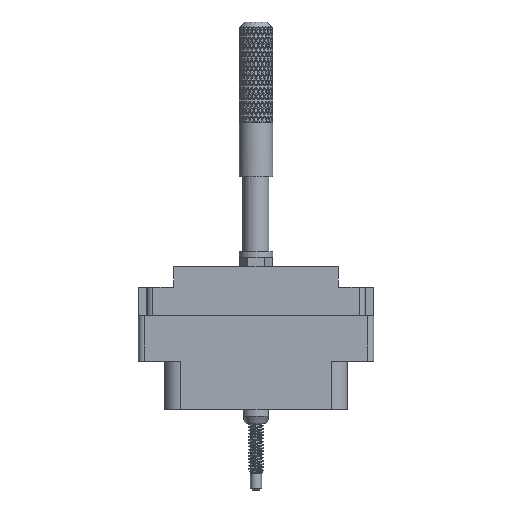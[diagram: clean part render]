
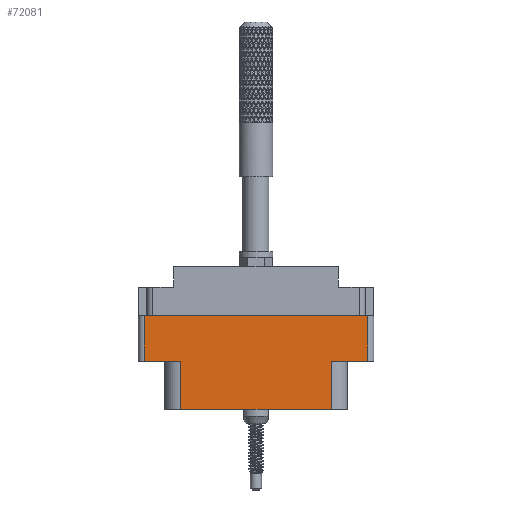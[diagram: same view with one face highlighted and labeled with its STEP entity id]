
A CAD part, front view. The second image highlights one B-rep face of the part: STEP entity #72081.
In plain terms, the highlighted planar face has unit normal (0, -1, 0).
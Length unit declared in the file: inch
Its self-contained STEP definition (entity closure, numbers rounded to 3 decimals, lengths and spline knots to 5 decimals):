
#5053 = CARTESIAN_POINT ( 'NONE',  ( -0.624, -0.343, -0.798 ) ) ;
#5832 = CARTESIAN_POINT ( 'NONE',  ( 0., -0.343, -0.274 ) ) ;
#7394 = ORIENTED_EDGE ( 'NONE', *, *, #25610, .T. ) ;
#9197 = DIRECTION ( 'NONE',  ( 0., 0., 1. ) ) ;
#9800 = CARTESIAN_POINT ( 'NONE',  ( 0.42052, -0.343, -0.529 ) ) ;
#10342 = EDGE_CURVE ( 'NONE', #183956, #45359, #106968, .T. ) ;
#12614 = VERTEX_POINT ( 'NONE', #67093 ) ;
#13844 = EDGE_LOOP ( 'NONE', ( #74284, #50483, #7394, #42640, #83809, #131305, #63630, #53074 ) ) ;
#14874 = CARTESIAN_POINT ( 'NONE',  ( -0.624, -0.343, -0.529 ) ) ;
#17578 = VECTOR ( 'NONE', #175656, 39.37008 ) ;
#25610 = EDGE_CURVE ( 'NONE', #47347, #115442, #118618, .T. ) ;
#26734 = CARTESIAN_POINT ( 'NONE',  ( 0., -0.343, -0.529 ) ) ;
#30810 = VECTOR ( 'NONE', #106284, 39.37008 ) ;
#31004 = EDGE_CURVE ( 'NONE', #85767, #45359, #68636, .T. ) ;
#31301 = EDGE_CURVE ( 'NONE', #85767, #79751, #117547, .T. ) ;
#37114 = LINE ( 'NONE', #5053, #135128 ) ;
#38152 = PLANE ( 'NONE',  #183256 ) ;
#42640 = ORIENTED_EDGE ( 'NONE', *, *, #184226, .T. ) ;
#45359 = VERTEX_POINT ( 'NONE', #67871 ) ;
#47347 = VERTEX_POINT ( 'NONE', #14874 ) ;
#50483 = ORIENTED_EDGE ( 'NONE', *, *, #165754, .T. ) ;
#53074 = ORIENTED_EDGE ( 'NONE', *, *, #31301, .T. ) ;
#55457 = DIRECTION ( 'NONE',  ( 0., 0., -1. ) ) ;
#63083 = LINE ( 'NONE', #169598, #67506 ) ;
#63630 = ORIENTED_EDGE ( 'NONE', *, *, #31004, .F. ) ;
#67093 = CARTESIAN_POINT ( 'NONE',  ( -0.42052, -0.343, -0.798 ) ) ;
#67506 = VECTOR ( 'NONE', #142862, 39.37008 ) ;
#67871 = CARTESIAN_POINT ( 'NONE',  ( 0.42052, -0.343, -0.529 ) ) ;
#68636 = LINE ( 'NONE', #26734, #130964 ) ;
#72081 = ADVANCED_FACE ( 'NONE', ( #176916 ), #38152, .T. ) ;
#73394 = EDGE_CURVE ( 'NONE', #12614, #183956, #63083, .T. ) ;
#74284 = ORIENTED_EDGE ( 'NONE', *, *, #77099, .F. ) ;
#77099 = EDGE_CURVE ( 'NONE', #117241, #79751, #171264, .T. ) ;
#77108 = CARTESIAN_POINT ( 'NONE',  ( -0.42052, -0.343, -0.798 ) ) ;
#79751 = VERTEX_POINT ( 'NONE', #93122 ) ;
#80774 = VECTOR ( 'NONE', #153478, 39.37008 ) ;
#83809 = ORIENTED_EDGE ( 'NONE', *, *, #73394, .T. ) ;
#85767 = VERTEX_POINT ( 'NONE', #97242 ) ;
#89193 = VECTOR ( 'NONE', #9197, 39.37008 ) ;
#93122 = CARTESIAN_POINT ( 'NONE',  ( 0.624, -0.343, -0.274 ) ) ;
#97242 = CARTESIAN_POINT ( 'NONE',  ( 0.624, -0.343, -0.529 ) ) ;
#99439 = DIRECTION ( 'NONE',  ( -1., 0., 0. ) ) ;
#99551 = CARTESIAN_POINT ( 'NONE',  ( -0.656, -0.343, -0.798 ) ) ;
#105735 = DIRECTION ( 'NONE',  ( 0., 0., -1. ) ) ;
#106284 = DIRECTION ( 'NONE',  ( 0., 0., 1. ) ) ;
#106968 = LINE ( 'NONE', #9800, #89193 ) ;
#107718 = VECTOR ( 'NONE', #105735, 39.37008 ) ;
#112680 = DIRECTION ( 'NONE',  ( 0., -1., 0. ) ) ;
#115442 = VERTEX_POINT ( 'NONE', #175873 ) ;
#117241 = VERTEX_POINT ( 'NONE', #154366 ) ;
#117547 = LINE ( 'NONE', #178413, #30810 ) ;
#118618 = LINE ( 'NONE', #183948, #80774 ) ;
#130964 = VECTOR ( 'NONE', #99439, 39.37008 ) ;
#131305 = ORIENTED_EDGE ( 'NONE', *, *, #10342, .T. ) ;
#135128 = VECTOR ( 'NONE', #159968, 39.37008 ) ;
#142862 = DIRECTION ( 'NONE',  ( 1., 0., 0. ) ) ;
#153478 = DIRECTION ( 'NONE',  ( 1., 0., 0. ) ) ;
#154366 = CARTESIAN_POINT ( 'NONE',  ( -0.624, -0.343, -0.274 ) ) ;
#159968 = DIRECTION ( 'NONE',  ( 0., 0., -1. ) ) ;
#165754 = EDGE_CURVE ( 'NONE', #117241, #47347, #37114, .T. ) ;
#166804 = CARTESIAN_POINT ( 'NONE',  ( 0.42052, -0.343, -0.798 ) ) ;
#169598 = CARTESIAN_POINT ( 'NONE',  ( -0.656, -0.343, -0.798 ) ) ;
#171264 = LINE ( 'NONE', #5832, #17578 ) ;
#174460 = LINE ( 'NONE', #77108, #107718 ) ;
#175656 = DIRECTION ( 'NONE',  ( 1., 0., 0. ) ) ;
#175873 = CARTESIAN_POINT ( 'NONE',  ( -0.42052, -0.343, -0.529 ) ) ;
#176916 = FACE_OUTER_BOUND ( 'NONE', #13844, .T. ) ;
#178413 = CARTESIAN_POINT ( 'NONE',  ( 0.624, -0.343, -0.798 ) ) ;
#183256 = AXIS2_PLACEMENT_3D ( 'NONE', #99551, #112680, #55457 ) ;
#183948 = CARTESIAN_POINT ( 'NONE',  ( 0., -0.343, -0.529 ) ) ;
#183956 = VERTEX_POINT ( 'NONE', #166804 ) ;
#184226 = EDGE_CURVE ( 'NONE', #115442, #12614, #174460, .T. ) ;
